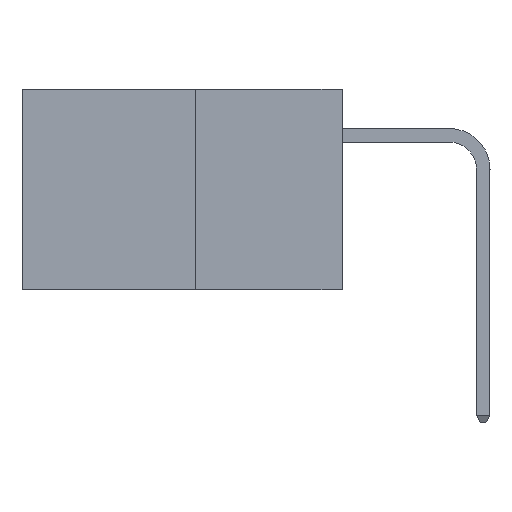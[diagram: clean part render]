
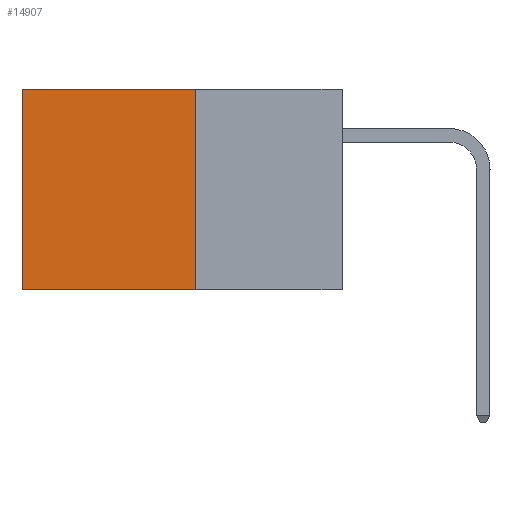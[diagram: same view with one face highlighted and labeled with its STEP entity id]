
A CAD part, left-side view. The second image highlights one B-rep face of the part: STEP entity #14907.
In plain terms, the highlighted planar face has unit normal (-1, 0, 0).
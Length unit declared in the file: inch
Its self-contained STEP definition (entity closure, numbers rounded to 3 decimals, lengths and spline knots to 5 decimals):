
#2176 = EDGE_LOOP ( 'NONE', ( #28252, #3671, #26062, #23955 ) ) ;
#3375 = VERTEX_POINT ( 'NONE', #13913 ) ;
#3399 = CARTESIAN_POINT ( 'NONE',  ( 0.277, 0.27, -0.37 ) ) ;
#3634 = VECTOR ( 'NONE', #25707, 39.37008 ) ;
#3671 = ORIENTED_EDGE ( 'NONE', *, *, #22820, .F. ) ;
#7380 = VERTEX_POINT ( 'NONE', #17199 ) ;
#9423 = VERTEX_POINT ( 'NONE', #25660 ) ;
#10512 = DIRECTION ( 'NONE',  ( 1., 0., 0. ) ) ;
#12629 = EDGE_CURVE ( 'NONE', #7380, #13213, #20665, .T. ) ;
#12753 = DIRECTION ( 'NONE',  ( 0., 1., 0. ) ) ;
#13213 = VERTEX_POINT ( 'NONE', #3399 ) ;
#13913 = CARTESIAN_POINT ( 'NONE',  ( 0.277, 0.59, -0.37 ) ) ;
#14492 = AXIS2_PLACEMENT_3D ( 'NONE', #25798, #10512, #28304 ) ;
#14551 = LINE ( 'NONE', #30425, #27267 ) ;
#14907 = ADVANCED_FACE ( 'NONE', ( #21689 ), #23264, .F. ) ;
#17127 = VECTOR ( 'NONE', #19132, 39.37008 ) ;
#17199 = CARTESIAN_POINT ( 'NONE',  ( 0.277, 0.27, 0. ) ) ;
#19132 = DIRECTION ( 'NONE',  ( 0., 1., 0. ) ) ;
#20665 = LINE ( 'NONE', #31751, #27378 ) ;
#21689 = FACE_OUTER_BOUND ( 'NONE', #2176, .T. ) ;
#22820 = EDGE_CURVE ( 'NONE', #13213, #3375, #23120, .T. ) ;
#23120 = LINE ( 'NONE', #24251, #17127 ) ;
#23170 = CARTESIAN_POINT ( 'NONE',  ( 0.277, 0.59, -0.37 ) ) ;
#23264 = PLANE ( 'NONE',  #14492 ) ;
#23955 = ORIENTED_EDGE ( 'NONE', *, *, #27469, .T. ) ;
#24251 = CARTESIAN_POINT ( 'NONE',  ( 0.277, 0.27, -0.37 ) ) ;
#25660 = CARTESIAN_POINT ( 'NONE',  ( 0.277, 0.59, 0. ) ) ;
#25707 = DIRECTION ( 'NONE',  ( 0., 0., -1. ) ) ;
#25798 = CARTESIAN_POINT ( 'NONE',  ( 0.277, 0.27, -0.37 ) ) ;
#26062 = ORIENTED_EDGE ( 'NONE', *, *, #12629, .F. ) ;
#26624 = EDGE_CURVE ( 'NONE', #9423, #3375, #29918, .T. ) ;
#27267 = VECTOR ( 'NONE', #12753, 39.37008 ) ;
#27378 = VECTOR ( 'NONE', #29186, 39.37008 ) ;
#27469 = EDGE_CURVE ( 'NONE', #7380, #9423, #14551, .T. ) ;
#28252 = ORIENTED_EDGE ( 'NONE', *, *, #26624, .T. ) ;
#28304 = DIRECTION ( 'NONE',  ( 0., 0., -1. ) ) ;
#29186 = DIRECTION ( 'NONE',  ( 0., 0., -1. ) ) ;
#29918 = LINE ( 'NONE', #23170, #3634 ) ;
#30425 = CARTESIAN_POINT ( 'NONE',  ( 0.277, 0.27, 0. ) ) ;
#31751 = CARTESIAN_POINT ( 'NONE',  ( 0.277, 0.27, -0.37 ) ) ;
